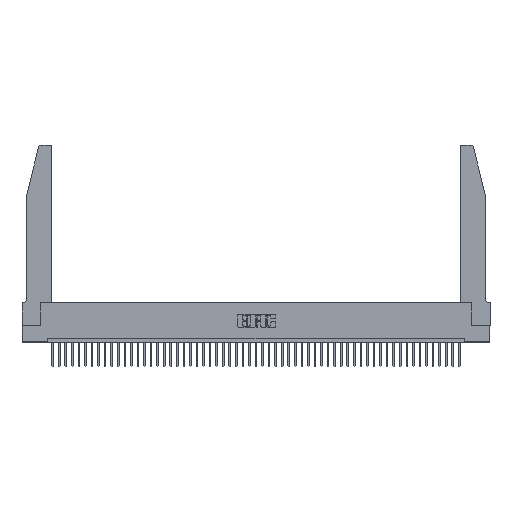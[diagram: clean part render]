
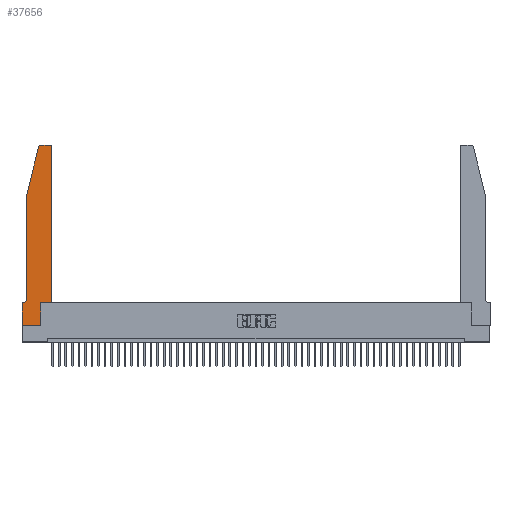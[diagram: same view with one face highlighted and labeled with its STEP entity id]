
A CAD part, top view. The second image highlights one B-rep face of the part: STEP entity #37656.
In plain terms, the highlighted planar face has unit normal (0, 0, 1).
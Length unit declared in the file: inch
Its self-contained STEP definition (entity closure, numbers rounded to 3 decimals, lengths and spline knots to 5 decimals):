
#174 = EDGE_CURVE ( 'NONE', #20997, #40942, #41066, .T. ) ;
#1345 = CARTESIAN_POINT ( 'NONE',  ( 0.0755, 2., 0.37 ) ) ;
#2138 = EDGE_CURVE ( 'NONE', #42154, #32051, #12855, .T. ) ;
#3104 = FACE_OUTER_BOUND ( 'NONE', #22665, .T. ) ;
#3401 = CARTESIAN_POINT ( 'NONE',  ( 0., 0., 0.37 ) ) ;
#3484 = CIRCLE ( 'NONE', #22950, 0.03 ) ;
#3650 = VERTEX_POINT ( 'NONE', #41822 ) ;
#4443 = CARTESIAN_POINT ( 'NONE',  ( 0.2865, 0., 0.37 ) ) ;
#4719 = LINE ( 'NONE', #25250, #8890 ) ;
#5211 = DIRECTION ( 'NONE',  ( 1., 0., 0. ) ) ;
#7956 = LINE ( 'NONE', #40848, #40888 ) ;
#8375 = VECTOR ( 'NONE', #22614, 39.37008 ) ;
#8506 = CARTESIAN_POINT ( 'NONE',  ( 0.284, 2.72, 0.37 ) ) ;
#8890 = VECTOR ( 'NONE', #29079, 39.37008 ) ;
#8905 = VERTEX_POINT ( 'NONE', #35975 ) ;
#9300 = DIRECTION ( 'NONE',  ( 0., 0., -1. ) ) ;
#10037 = EDGE_CURVE ( 'NONE', #3650, #18958, #45791, .T. ) ;
#11206 = VECTOR ( 'NONE', #12169, 39.37008 ) ;
#12169 = DIRECTION ( 'NONE',  ( 0., -1., 0. ) ) ;
#12207 = CARTESIAN_POINT ( 'NONE',  ( 0., 0., 0.37 ) ) ;
#12226 = VECTOR ( 'NONE', #48120, 39.37008 ) ;
#12358 = DIRECTION ( 'NONE',  ( 0., 0., 1. ) ) ;
#12833 = CARTESIAN_POINT ( 'NONE',  ( 0.4205, 2.75, 0.37 ) ) ;
#12855 = LINE ( 'NONE', #40742, #26610 ) ;
#12939 = VECTOR ( 'NONE', #30252, 39.37008 ) ;
#13368 = DIRECTION ( 'NONE',  ( 1., 0., 0. ) ) ;
#14089 = DIRECTION ( 'NONE',  ( 1., 0., 0. ) ) ;
#16105 = ORIENTED_EDGE ( 'NONE', *, *, #2138, .T. ) ;
#16504 = EDGE_CURVE ( 'NONE', #18958, #46108, #46282, .T. ) ;
#16641 = CARTESIAN_POINT ( 'NONE',  ( 0., 0.35, 0.37 ) ) ;
#17875 = VECTOR ( 'NONE', #40264, 39.37008 ) ;
#17882 = CARTESIAN_POINT ( 'NONE',  ( 0.0755, 2., 0.37 ) ) ;
#17928 = EDGE_CURVE ( 'NONE', #48379, #8905, #7956, .T. ) ;
#18674 = EDGE_CURVE ( 'NONE', #32051, #42309, #33647, .T. ) ;
#18958 = VERTEX_POINT ( 'NONE', #36076 ) ;
#19156 = EDGE_CURVE ( 'NONE', #8905, #29557, #30314, .T. ) ;
#20997 = VERTEX_POINT ( 'NONE', #16641 ) ;
#21214 = CARTESIAN_POINT ( 'NONE',  ( 0.4205, 2.72, 0.37 ) ) ;
#21422 = CARTESIAN_POINT ( 'NONE',  ( 0.4505, 0.35, 0.37 ) ) ;
#22614 = DIRECTION ( 'NONE',  ( -1., 0., 0. ) ) ;
#22665 = EDGE_LOOP ( 'NONE', ( #16105, #26092, #24017, #33098, #41386, #34994, #23865, #43833, #31008, #38286, #36500, #49064 ) ) ;
#22905 = PLANE ( 'NONE',  #46346 ) ;
#22950 = AXIS2_PLACEMENT_3D ( 'NONE', #21214, #43920, #13368 ) ;
#23865 = ORIENTED_EDGE ( 'NONE', *, *, #174, .T. ) ;
#24017 = ORIENTED_EDGE ( 'NONE', *, *, #45133, .T. ) ;
#25250 = CARTESIAN_POINT ( 'NONE',  ( 0.4505, 0.35, 0.37 ) ) ;
#25713 = CARTESIAN_POINT ( 'NONE',  ( 0.25487, 2.72718, 0.37 ) ) ;
#25910 = CARTESIAN_POINT ( 'NONE',  ( 0., 0.35, 0.37 ) ) ;
#26092 = ORIENTED_EDGE ( 'NONE', *, *, #18674, .T. ) ;
#26610 = VECTOR ( 'NONE', #44574, 39.37008 ) ;
#29079 = DIRECTION ( 'NONE',  ( 0., 1., 0. ) ) ;
#29285 = DIRECTION ( 'NONE',  ( 0., 0., 1. ) ) ;
#29557 = VERTEX_POINT ( 'NONE', #21422 ) ;
#30252 = DIRECTION ( 'NONE',  ( 0., -1., 0. ) ) ;
#30314 = LINE ( 'NONE', #43071, #42262 ) ;
#30360 = VERTEX_POINT ( 'NONE', #46636 ) ;
#31008 = ORIENTED_EDGE ( 'NONE', *, *, #17928, .T. ) ;
#31078 = LINE ( 'NONE', #41652, #8375 ) ;
#31361 = DIRECTION ( 'NONE',  ( 1., 0., 0. ) ) ;
#31688 = EDGE_CURVE ( 'NONE', #46108, #20997, #31078, .T. ) ;
#32003 = DIRECTION ( 'NONE',  ( -1., 0., 0. ) ) ;
#32051 = VERTEX_POINT ( 'NONE', #40373 ) ;
#32085 = AXIS2_PLACEMENT_3D ( 'NONE', #43345, #9300, #32003 ) ;
#33098 = ORIENTED_EDGE ( 'NONE', *, *, #10037, .T. ) ;
#33647 = CIRCLE ( 'NONE', #35651, 0.03 ) ;
#34994 = ORIENTED_EDGE ( 'NONE', *, *, #31688, .T. ) ;
#35651 = AXIS2_PLACEMENT_3D ( 'NONE', #8506, #12358, #5211 ) ;
#35975 = CARTESIAN_POINT ( 'NONE',  ( 0.2865, 0.35, 0.37 ) ) ;
#36076 = CARTESIAN_POINT ( 'NONE',  ( 0.0755, 0.42, 0.37 ) ) ;
#36500 = ORIENTED_EDGE ( 'NONE', *, *, #48055, .T. ) ;
#37656 = ADVANCED_FACE ( 'NONE', ( #3104 ), #22905, .T. ) ;
#38286 = ORIENTED_EDGE ( 'NONE', *, *, #19156, .T. ) ;
#40264 = DIRECTION ( 'NONE',  ( 1., 0., 0. ) ) ;
#40373 = CARTESIAN_POINT ( 'NONE',  ( 0.284, 2.75, 0.37 ) ) ;
#40742 = CARTESIAN_POINT ( 'NONE',  ( 0.2605, 2.75, 0.37 ) ) ;
#40848 = CARTESIAN_POINT ( 'NONE',  ( 0.2865, 0.35, 0.37 ) ) ;
#40888 = VECTOR ( 'NONE', #44012, 39.37008 ) ;
#40942 = VERTEX_POINT ( 'NONE', #12207 ) ;
#41066 = LINE ( 'NONE', #3401, #12939 ) ;
#41386 = ORIENTED_EDGE ( 'NONE', *, *, #16504, .T. ) ;
#41652 = CARTESIAN_POINT ( 'NONE',  ( 0.0755, 0.35, 0.37 ) ) ;
#41822 = CARTESIAN_POINT ( 'NONE',  ( 0.0755, 2., 0.37 ) ) ;
#42154 = VERTEX_POINT ( 'NONE', #12833 ) ;
#42262 = VECTOR ( 'NONE', #31361, 39.37008 ) ;
#42309 = VERTEX_POINT ( 'NONE', #25713 ) ;
#43071 = CARTESIAN_POINT ( 'NONE',  ( 0.4505, 0.35, 0.37 ) ) ;
#43345 = CARTESIAN_POINT ( 'NONE',  ( 0.0055, 0.42, 0.37 ) ) ;
#43739 = EDGE_CURVE ( 'NONE', #30360, #42154, #3484, .T. ) ;
#43771 = CARTESIAN_POINT ( 'NONE',  ( 0., 0., 0.37 ) ) ;
#43833 = ORIENTED_EDGE ( 'NONE', *, *, #47893, .T. ) ;
#43920 = DIRECTION ( 'NONE',  ( 0., 0., 1. ) ) ;
#44012 = DIRECTION ( 'NONE',  ( 0., 1., 0. ) ) ;
#44574 = DIRECTION ( 'NONE',  ( -1., 0., 0. ) ) ;
#45133 = EDGE_CURVE ( 'NONE', #42309, #3650, #48721, .T. ) ;
#45791 = LINE ( 'NONE', #1345, #11206 ) ;
#46108 = VERTEX_POINT ( 'NONE', #46622 ) ;
#46282 = CIRCLE ( 'NONE', #32085, 0.07 ) ;
#46346 = AXIS2_PLACEMENT_3D ( 'NONE', #25910, #29285, #14089 ) ;
#46622 = CARTESIAN_POINT ( 'NONE',  ( 0.0055, 0.35, 0.37 ) ) ;
#46636 = CARTESIAN_POINT ( 'NONE',  ( 0.4505, 2.72, 0.37 ) ) ;
#47893 = EDGE_CURVE ( 'NONE', #40942, #48379, #48376, .T. ) ;
#48055 = EDGE_CURVE ( 'NONE', #29557, #30360, #4719, .T. ) ;
#48120 = DIRECTION ( 'NONE',  ( -0.239, -0.971, 0. ) ) ;
#48376 = LINE ( 'NONE', #43771, #17875 ) ;
#48379 = VERTEX_POINT ( 'NONE', #4443 ) ;
#48721 = LINE ( 'NONE', #17882, #12226 ) ;
#49064 = ORIENTED_EDGE ( 'NONE', *, *, #43739, .T. ) ;
